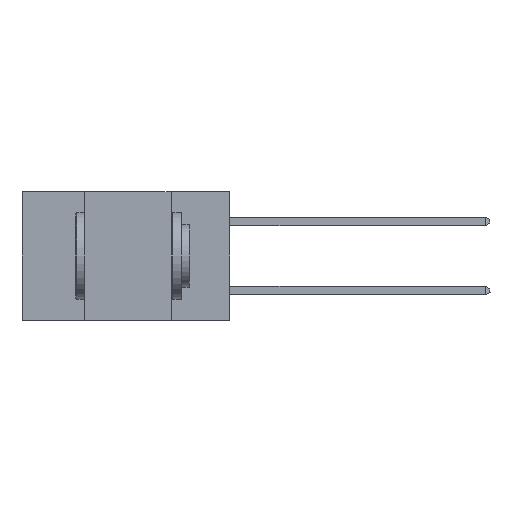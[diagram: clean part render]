
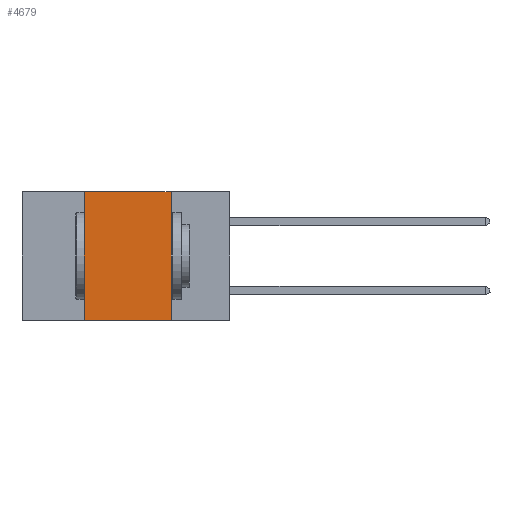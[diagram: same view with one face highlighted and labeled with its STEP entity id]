
A CAD part, left-side view. The second image highlights one B-rep face of the part: STEP entity #4679.
In plain terms, the highlighted planar face has unit normal (-1, 0, 0).
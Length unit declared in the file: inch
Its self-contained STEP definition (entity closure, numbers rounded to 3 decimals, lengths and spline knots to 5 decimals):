
#1126 = ORIENTED_EDGE ( 'NONE', *, *, #9853, .T. ) ;
#1497 = DIRECTION ( 'NONE',  ( 0., 0., -1. ) ) ;
#1653 = ORIENTED_EDGE ( 'NONE', *, *, #10749, .F. ) ;
#2278 = CARTESIAN_POINT ( 'NONE',  ( 0., 0.42, 0. ) ) ;
#2490 = VERTEX_POINT ( 'NONE', #3693 ) ;
#2564 = DIRECTION ( 'NONE',  ( 0., 0., -1. ) ) ;
#3156 = FACE_OUTER_BOUND ( 'NONE', #5162, .T. ) ;
#3285 = DIRECTION ( 'NONE',  ( 0., -1., 0. ) ) ;
#3693 = CARTESIAN_POINT ( 'NONE',  ( 0., 0.42, -0.37 ) ) ;
#3800 = VECTOR ( 'NONE', #11714, 39.37008 ) ;
#3985 = VECTOR ( 'NONE', #2564, 39.37008 ) ;
#4679 = ADVANCED_FACE ( 'NONE', ( #3156 ), #13480, .F. ) ;
#5162 = EDGE_LOOP ( 'NONE', ( #1653, #6534, #13181, #1126 ) ) ;
#5476 = LINE ( 'NONE', #12978, #15173 ) ;
#6534 = ORIENTED_EDGE ( 'NONE', *, *, #9467, .F. ) ;
#6749 = CARTESIAN_POINT ( 'NONE',  ( 0., 0.6, 0. ) ) ;
#7417 = VERTEX_POINT ( 'NONE', #7922 ) ;
#7784 = AXIS2_PLACEMENT_3D ( 'NONE', #11103, #8610, #1497 ) ;
#7922 = CARTESIAN_POINT ( 'NONE',  ( 0., 0.17, 0. ) ) ;
#8052 = CARTESIAN_POINT ( 'NONE',  ( 0., 0.42, 0. ) ) ;
#8587 = VECTOR ( 'NONE', #14387, 39.37008 ) ;
#8610 = DIRECTION ( 'NONE',  ( 1., 0., 0. ) ) ;
#9467 = EDGE_CURVE ( 'NONE', #12486, #7417, #11543, .T. ) ;
#9853 = EDGE_CURVE ( 'NONE', #2490, #11999, #5476, .T. ) ;
#10749 = EDGE_CURVE ( 'NONE', #7417, #11999, #11337, .T. ) ;
#11103 = CARTESIAN_POINT ( 'NONE',  ( 0., 0.6, 0. ) ) ;
#11337 = LINE ( 'NONE', #12183, #3985 ) ;
#11543 = LINE ( 'NONE', #6749, #3800 ) ;
#11714 = DIRECTION ( 'NONE',  ( 0., -1., 0. ) ) ;
#11999 = VERTEX_POINT ( 'NONE', #12494 ) ;
#12183 = CARTESIAN_POINT ( 'NONE',  ( 0., 0.17, 0. ) ) ;
#12486 = VERTEX_POINT ( 'NONE', #8052 ) ;
#12494 = CARTESIAN_POINT ( 'NONE',  ( 0., 0.17, -0.37 ) ) ;
#12978 = CARTESIAN_POINT ( 'NONE',  ( 0., 0.6, -0.37 ) ) ;
#13159 = EDGE_CURVE ( 'NONE', #2490, #12486, #15656, .T. ) ;
#13181 = ORIENTED_EDGE ( 'NONE', *, *, #13159, .F. ) ;
#13480 = PLANE ( 'NONE',  #7784 ) ;
#14387 = DIRECTION ( 'NONE',  ( 0., 0., 1. ) ) ;
#15173 = VECTOR ( 'NONE', #3285, 39.37008 ) ;
#15656 = LINE ( 'NONE', #2278, #8587 ) ;
